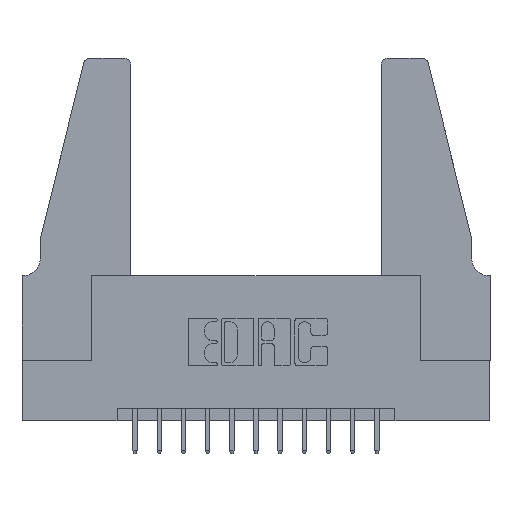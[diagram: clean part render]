
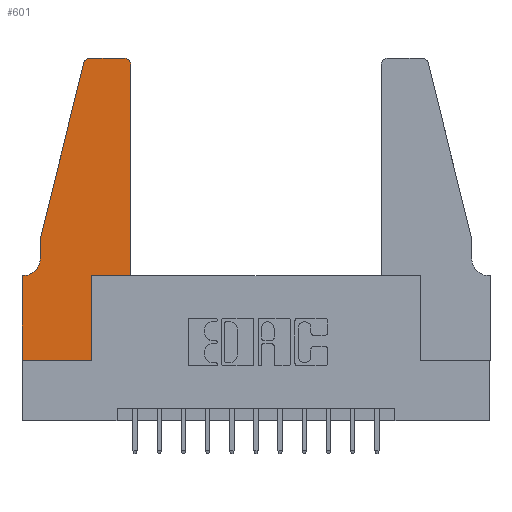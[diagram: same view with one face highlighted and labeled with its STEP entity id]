
A CAD part, top view. The second image highlights one B-rep face of the part: STEP entity #601.
In plain terms, the highlighted planar face has unit normal (0, 0, 1).
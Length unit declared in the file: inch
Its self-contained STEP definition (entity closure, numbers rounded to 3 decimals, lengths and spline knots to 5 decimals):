
#439 = VECTOR ( 'NONE', #3507, 39.37008 ) ;
#601 = ADVANCED_FACE ( 'NONE', ( #6992 ), #14953, .T. ) ;
#655 = VECTOR ( 'NONE', #13489, 39.37008 ) ;
#796 = DIRECTION ( 'NONE',  ( -0.239, -0.971, 0. ) ) ;
#1141 = EDGE_LOOP ( 'NONE', ( #3579, #10585, #8176, #12963, #4477, #2539, #5883, #11811, #4534, #12057, #12443, #7387 ) ) ;
#1187 = CARTESIAN_POINT ( 'NONE',  ( 0.4205, 1.25, 0.37 ) ) ;
#1288 = EDGE_CURVE ( 'NONE', #13387, #5235, #10683, .T. ) ;
#1319 = VERTEX_POINT ( 'NONE', #8344 ) ;
#1347 = CARTESIAN_POINT ( 'NONE',  ( 0.4205, 1.22, 0.37 ) ) ;
#1360 = LINE ( 'NONE', #10550, #3410 ) ;
#1599 = CARTESIAN_POINT ( 'NONE',  ( 0., 0.35, 0.37 ) ) ;
#2139 = DIRECTION ( 'NONE',  ( 0., 0., -1. ) ) ;
#2403 = VERTEX_POINT ( 'NONE', #14018 ) ;
#2467 = CARTESIAN_POINT ( 'NONE',  ( 0.4505, 0.35, 0.37 ) ) ;
#2539 = ORIENTED_EDGE ( 'NONE', *, *, #5138, .T. ) ;
#2626 = EDGE_CURVE ( 'NONE', #10472, #8169, #11367, .T. ) ;
#3092 = AXIS2_PLACEMENT_3D ( 'NONE', #10364, #5714, #4547 ) ;
#3134 = CIRCLE ( 'NONE', #10467, 0.07 ) ;
#3301 = CARTESIAN_POINT ( 'NONE',  ( 0.0755, 0.5, 0.37 ) ) ;
#3410 = VECTOR ( 'NONE', #4880, 39.37008 ) ;
#3507 = DIRECTION ( 'NONE',  ( 0., -1., 0. ) ) ;
#3546 = DIRECTION ( 'NONE',  ( 0., -1., 0. ) ) ;
#3579 = ORIENTED_EDGE ( 'NONE', *, *, #7865, .T. ) ;
#3868 = LINE ( 'NONE', #9837, #655 ) ;
#4013 = EDGE_CURVE ( 'NONE', #6738, #4362, #10837, .T. ) ;
#4362 = VERTEX_POINT ( 'NONE', #13240 ) ;
#4477 = ORIENTED_EDGE ( 'NONE', *, *, #12481, .T. ) ;
#4480 = EDGE_CURVE ( 'NONE', #5235, #1319, #6549, .T. ) ;
#4511 = CARTESIAN_POINT ( 'NONE',  ( 0., 0.35, 0.37 ) ) ;
#4534 = ORIENTED_EDGE ( 'NONE', *, *, #4480, .T. ) ;
#4547 = DIRECTION ( 'NONE',  ( 1., 0., 0. ) ) ;
#4659 = CARTESIAN_POINT ( 'NONE',  ( 0.0755, 0.5, 0.37 ) ) ;
#4880 = DIRECTION ( 'NONE',  ( -1., 0., 0. ) ) ;
#5138 = EDGE_CURVE ( 'NONE', #2403, #13950, #1360, .T. ) ;
#5235 = VERTEX_POINT ( 'NONE', #9932 ) ;
#5714 = DIRECTION ( 'NONE',  ( 0., 0., 1. ) ) ;
#5883 = ORIENTED_EDGE ( 'NONE', *, *, #13653, .T. ) ;
#6045 = DIRECTION ( 'NONE',  ( 0., 0., 1. ) ) ;
#6549 = LINE ( 'NONE', #12429, #12231 ) ;
#6738 = VERTEX_POINT ( 'NONE', #2467 ) ;
#6992 = FACE_OUTER_BOUND ( 'NONE', #1141, .T. ) ;
#7136 = VECTOR ( 'NONE', #11607, 39.37008 ) ;
#7263 = CARTESIAN_POINT ( 'NONE',  ( 0., 0., 0.37 ) ) ;
#7343 = VECTOR ( 'NONE', #13746, 39.37008 ) ;
#7387 = ORIENTED_EDGE ( 'NONE', *, *, #14250, .T. ) ;
#7865 = EDGE_CURVE ( 'NONE', #13605, #14048, #12707, .T. ) ;
#8169 = VERTEX_POINT ( 'NONE', #8600 ) ;
#8176 = ORIENTED_EDGE ( 'NONE', *, *, #2626, .T. ) ;
#8232 = CIRCLE ( 'NONE', #8466, 0.03 ) ;
#8344 = CARTESIAN_POINT ( 'NONE',  ( 0.2865, 0.35, 0.37 ) ) ;
#8466 = AXIS2_PLACEMENT_3D ( 'NONE', #1347, #6045, #10693 ) ;
#8600 = CARTESIAN_POINT ( 'NONE',  ( 0.0755, 0.5, 0.37 ) ) ;
#8847 = DIRECTION ( 'NONE',  ( 0., 1., 0. ) ) ;
#8986 = DIRECTION ( 'NONE',  ( 0., 0., 1. ) ) ;
#9123 = CARTESIAN_POINT ( 'NONE',  ( 0.2605, 1.25, 0.37 ) ) ;
#9200 = DIRECTION ( 'NONE',  ( 1., 0., 0. ) ) ;
#9549 = EDGE_CURVE ( 'NONE', #1319, #6738, #3868, .T. ) ;
#9644 = CARTESIAN_POINT ( 'NONE',  ( 0.284, 1.25, 0.37 ) ) ;
#9656 = EDGE_CURVE ( 'NONE', #14048, #10472, #9703, .T. ) ;
#9703 = CIRCLE ( 'NONE', #3092, 0.03 ) ;
#9778 = VECTOR ( 'NONE', #12140, 39.37008 ) ;
#9837 = CARTESIAN_POINT ( 'NONE',  ( 0.4505, 0.35, 0.37 ) ) ;
#9932 = CARTESIAN_POINT ( 'NONE',  ( 0.2865, 0., 0.37 ) ) ;
#10364 = CARTESIAN_POINT ( 'NONE',  ( 0.284, 1.22, 0.37 ) ) ;
#10448 = VERTEX_POINT ( 'NONE', #12869 ) ;
#10467 = AXIS2_PLACEMENT_3D ( 'NONE', #14760, #2139, #13703 ) ;
#10472 = VERTEX_POINT ( 'NONE', #13758 ) ;
#10550 = CARTESIAN_POINT ( 'NONE',  ( 0.0755, 0.35, 0.37 ) ) ;
#10585 = ORIENTED_EDGE ( 'NONE', *, *, #9656, .T. ) ;
#10683 = LINE ( 'NONE', #7263, #7136 ) ;
#10693 = DIRECTION ( 'NONE',  ( 1., 0., 0. ) ) ;
#10837 = LINE ( 'NONE', #13109, #9778 ) ;
#11367 = LINE ( 'NONE', #3301, #13471 ) ;
#11574 = LINE ( 'NONE', #4659, #439 ) ;
#11607 = DIRECTION ( 'NONE',  ( 1., 0., 0. ) ) ;
#11811 = ORIENTED_EDGE ( 'NONE', *, *, #1288, .T. ) ;
#12027 = AXIS2_PLACEMENT_3D ( 'NONE', #4511, #8986, #9200 ) ;
#12057 = ORIENTED_EDGE ( 'NONE', *, *, #9549, .T. ) ;
#12140 = DIRECTION ( 'NONE',  ( 0., 1., 0. ) ) ;
#12231 = VECTOR ( 'NONE', #8847, 39.37008 ) ;
#12429 = CARTESIAN_POINT ( 'NONE',  ( 0.2865, 0.35, 0.37 ) ) ;
#12443 = ORIENTED_EDGE ( 'NONE', *, *, #4013, .T. ) ;
#12481 = EDGE_CURVE ( 'NONE', #10448, #2403, #3134, .T. ) ;
#12707 = LINE ( 'NONE', #9123, #7343 ) ;
#12863 = EDGE_CURVE ( 'NONE', #8169, #10448, #11574, .T. ) ;
#12869 = CARTESIAN_POINT ( 'NONE',  ( 0.0755, 0.42, 0.37 ) ) ;
#12963 = ORIENTED_EDGE ( 'NONE', *, *, #12863, .T. ) ;
#13109 = CARTESIAN_POINT ( 'NONE',  ( 0.4505, 0.35, 0.37 ) ) ;
#13205 = CARTESIAN_POINT ( 'NONE',  ( 0., 0., 0.37 ) ) ;
#13240 = CARTESIAN_POINT ( 'NONE',  ( 0.4505, 1.22, 0.37 ) ) ;
#13387 = VERTEX_POINT ( 'NONE', #13205 ) ;
#13471 = VECTOR ( 'NONE', #796, 39.37008 ) ;
#13489 = DIRECTION ( 'NONE',  ( 1., 0., 0. ) ) ;
#13605 = VERTEX_POINT ( 'NONE', #1187 ) ;
#13653 = EDGE_CURVE ( 'NONE', #13950, #13387, #13940, .T. ) ;
#13703 = DIRECTION ( 'NONE',  ( -1., 0., 0. ) ) ;
#13746 = DIRECTION ( 'NONE',  ( -1., 0., 0. ) ) ;
#13758 = CARTESIAN_POINT ( 'NONE',  ( 0.25487, 1.22718, 0.37 ) ) ;
#13765 = VECTOR ( 'NONE', #3546, 39.37008 ) ;
#13940 = LINE ( 'NONE', #14923, #13765 ) ;
#13950 = VERTEX_POINT ( 'NONE', #1599 ) ;
#14018 = CARTESIAN_POINT ( 'NONE',  ( 0.0055, 0.35, 0.37 ) ) ;
#14048 = VERTEX_POINT ( 'NONE', #9644 ) ;
#14250 = EDGE_CURVE ( 'NONE', #4362, #13605, #8232, .T. ) ;
#14760 = CARTESIAN_POINT ( 'NONE',  ( 0.0055, 0.42, 0.37 ) ) ;
#14923 = CARTESIAN_POINT ( 'NONE',  ( 0., 0., 0.37 ) ) ;
#14953 = PLANE ( 'NONE',  #12027 ) ;
